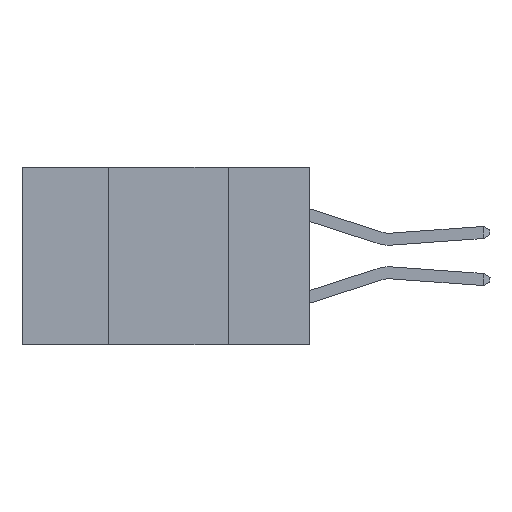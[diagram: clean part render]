
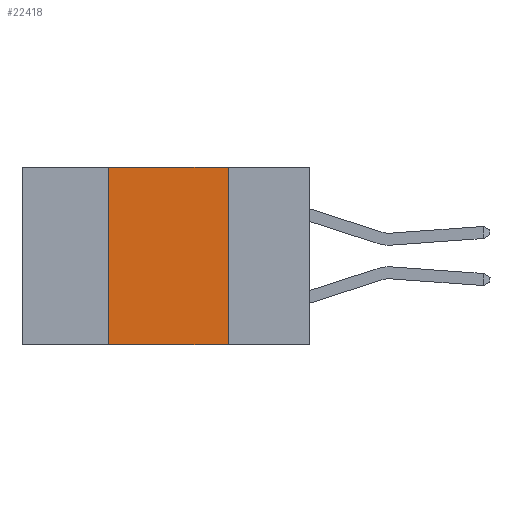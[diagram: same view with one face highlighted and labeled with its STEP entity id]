
A CAD part, left-side view. The second image highlights one B-rep face of the part: STEP entity #22418.
In plain terms, the highlighted planar face has unit normal (-1, 0, 0).
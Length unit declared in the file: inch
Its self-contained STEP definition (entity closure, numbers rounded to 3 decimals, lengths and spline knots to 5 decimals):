
#66 = VECTOR ( 'NONE', #7999, 39.37008 ) ;
#1132 = CARTESIAN_POINT ( 'NONE',  ( 0., 0.6, -0.37 ) ) ;
#1756 = VERTEX_POINT ( 'NONE', #23555 ) ;
#1838 = EDGE_LOOP ( 'NONE', ( #17741, #2163, #17136, #6776 ) ) ;
#2068 = CARTESIAN_POINT ( 'NONE',  ( 0., 0.6, 0. ) ) ;
#2163 = ORIENTED_EDGE ( 'NONE', *, *, #11175, .F. ) ;
#3104 = DIRECTION ( 'NONE',  ( 0., -1., 0. ) ) ;
#3172 = CARTESIAN_POINT ( 'NONE',  ( 0., 0.42, -0.37 ) ) ;
#3455 = VERTEX_POINT ( 'NONE', #5975 ) ;
#4674 = LINE ( 'NONE', #2068, #66 ) ;
#5222 = DIRECTION ( 'NONE',  ( 1., 0., 0. ) ) ;
#5558 = CARTESIAN_POINT ( 'NONE',  ( 0., 0.42, 0. ) ) ;
#5975 = CARTESIAN_POINT ( 'NONE',  ( 0., 0.17, -0.37 ) ) ;
#6776 = ORIENTED_EDGE ( 'NONE', *, *, #21709, .T. ) ;
#7418 = VECTOR ( 'NONE', #21445, 39.37008 ) ;
#7999 = DIRECTION ( 'NONE',  ( 0., -1., 0. ) ) ;
#9089 = DIRECTION ( 'NONE',  ( 0., 0., 1. ) ) ;
#11175 = EDGE_CURVE ( 'NONE', #15925, #1756, #4674, .T. ) ;
#13042 = FACE_OUTER_BOUND ( 'NONE', #1838, .T. ) ;
#13414 = CARTESIAN_POINT ( 'NONE',  ( 0., 0.42, -0.37 ) ) ;
#14717 = VERTEX_POINT ( 'NONE', #13414 ) ;
#15204 = EDGE_CURVE ( 'NONE', #14717, #15925, #20962, .T. ) ;
#15925 = VERTEX_POINT ( 'NONE', #5558 ) ;
#16908 = CARTESIAN_POINT ( 'NONE',  ( 0., 0.6, 0. ) ) ;
#17136 = ORIENTED_EDGE ( 'NONE', *, *, #15204, .F. ) ;
#17741 = ORIENTED_EDGE ( 'NONE', *, *, #19581, .F. ) ;
#17757 = LINE ( 'NONE', #19510, #7418 ) ;
#18386 = AXIS2_PLACEMENT_3D ( 'NONE', #16908, #5222, #18865 ) ;
#18865 = DIRECTION ( 'NONE',  ( 0., 0., -1. ) ) ;
#19510 = CARTESIAN_POINT ( 'NONE',  ( 0., 0.17, -0.37 ) ) ;
#19581 = EDGE_CURVE ( 'NONE', #1756, #3455, #17757, .T. ) ;
#20356 = VECTOR ( 'NONE', #9089, 39.37008 ) ;
#20962 = LINE ( 'NONE', #3172, #20356 ) ;
#20967 = VECTOR ( 'NONE', #3104, 39.37008 ) ;
#21445 = DIRECTION ( 'NONE',  ( 0., 0., -1. ) ) ;
#21709 = EDGE_CURVE ( 'NONE', #14717, #3455, #24865, .T. ) ;
#22418 = ADVANCED_FACE ( 'NONE', ( #13042 ), #22634, .F. ) ;
#22634 = PLANE ( 'NONE',  #18386 ) ;
#23555 = CARTESIAN_POINT ( 'NONE',  ( 0., 0.17, 0. ) ) ;
#24865 = LINE ( 'NONE', #1132, #20967 ) ;
